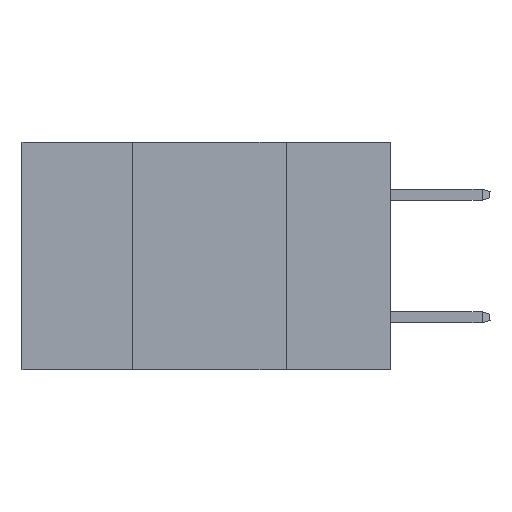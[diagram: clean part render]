
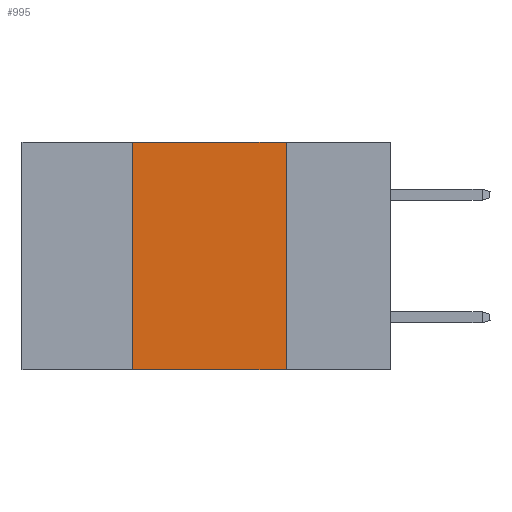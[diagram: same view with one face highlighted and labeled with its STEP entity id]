
A CAD part, left-side view. The second image highlights one B-rep face of the part: STEP entity #995.
In plain terms, the highlighted planar face has unit normal (-1, 0, 0).
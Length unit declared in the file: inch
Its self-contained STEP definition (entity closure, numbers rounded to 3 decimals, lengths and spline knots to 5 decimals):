
#995 = ADVANCED_FACE ( 'NONE', ( #3007 ), #7113, .F. ) ;
#1461 = LINE ( 'NONE', #6529, #9150 ) ;
#1471 = VECTOR ( 'NONE', #12758, 39.37008 ) ;
#2158 = AXIS2_PLACEMENT_3D ( 'NONE', #5635, #10111, #2420 ) ;
#2259 = ORIENTED_EDGE ( 'NONE', *, *, #7597, .F. ) ;
#2420 = DIRECTION ( 'NONE',  ( 0., 0., -1. ) ) ;
#2748 = VERTEX_POINT ( 'NONE', #7261 ) ;
#2788 = EDGE_CURVE ( 'NONE', #10734, #6264, #10369, .T. ) ;
#2809 = VECTOR ( 'NONE', #4181, 39.37008 ) ;
#3007 = FACE_OUTER_BOUND ( 'NONE', #10044, .T. ) ;
#3908 = CARTESIAN_POINT ( 'NONE',  ( 0., 0.42, -0.37 ) ) ;
#4181 = DIRECTION ( 'NONE',  ( 0., -1., 0. ) ) ;
#4192 = LINE ( 'NONE', #6948, #1471 ) ;
#4943 = ORIENTED_EDGE ( 'NONE', *, *, #7080, .F. ) ;
#5492 = VERTEX_POINT ( 'NONE', #10178 ) ;
#5635 = CARTESIAN_POINT ( 'NONE',  ( 0., 0.6, 0. ) ) ;
#6264 = VERTEX_POINT ( 'NONE', #8468 ) ;
#6529 = CARTESIAN_POINT ( 'NONE',  ( 0., 0.42, 0. ) ) ;
#6948 = CARTESIAN_POINT ( 'NONE',  ( 0., 0.17, 0. ) ) ;
#7080 = EDGE_CURVE ( 'NONE', #5492, #2748, #7543, .T. ) ;
#7113 = PLANE ( 'NONE',  #2158 ) ;
#7261 = CARTESIAN_POINT ( 'NONE',  ( 0., 0.17, 0. ) ) ;
#7521 = CARTESIAN_POINT ( 'NONE',  ( 0., 0.6, -0.37 ) ) ;
#7543 = LINE ( 'NONE', #10146, #2809 ) ;
#7597 = EDGE_CURVE ( 'NONE', #2748, #6264, #4192, .T. ) ;
#7662 = ORIENTED_EDGE ( 'NONE', *, *, #12876, .F. ) ;
#8468 = CARTESIAN_POINT ( 'NONE',  ( 0., 0.17, -0.37 ) ) ;
#9150 = VECTOR ( 'NONE', #11367, 39.37008 ) ;
#9294 = DIRECTION ( 'NONE',  ( 0., -1., 0. ) ) ;
#10044 = EDGE_LOOP ( 'NONE', ( #2259, #4943, #7662, #12729 ) ) ;
#10093 = VECTOR ( 'NONE', #9294, 39.37008 ) ;
#10111 = DIRECTION ( 'NONE',  ( 1., 0., 0. ) ) ;
#10146 = CARTESIAN_POINT ( 'NONE',  ( 0., 0.6, 0. ) ) ;
#10178 = CARTESIAN_POINT ( 'NONE',  ( 0., 0.42, 0. ) ) ;
#10369 = LINE ( 'NONE', #7521, #10093 ) ;
#10734 = VERTEX_POINT ( 'NONE', #3908 ) ;
#11367 = DIRECTION ( 'NONE',  ( 0., 0., 1. ) ) ;
#12729 = ORIENTED_EDGE ( 'NONE', *, *, #2788, .T. ) ;
#12758 = DIRECTION ( 'NONE',  ( 0., 0., -1. ) ) ;
#12876 = EDGE_CURVE ( 'NONE', #10734, #5492, #1461, .T. ) ;
